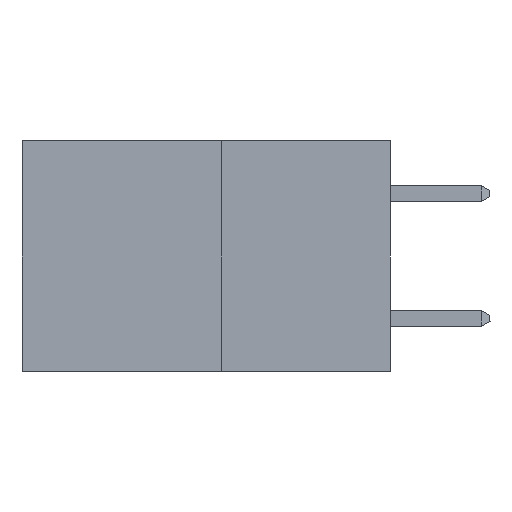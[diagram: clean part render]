
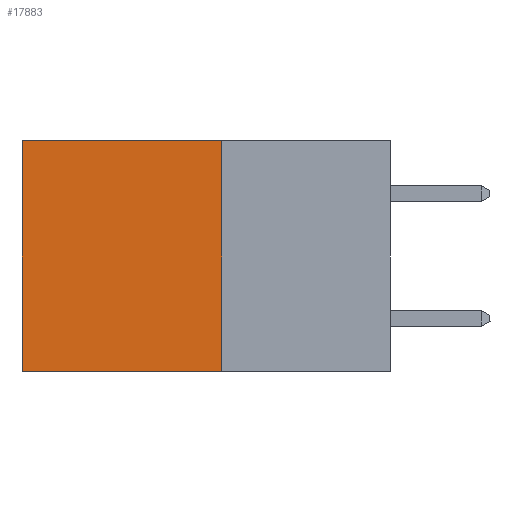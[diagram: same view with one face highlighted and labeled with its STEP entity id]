
A CAD part, left-side view. The second image highlights one B-rep face of the part: STEP entity #17883.
In plain terms, the highlighted planar face has unit normal (-1, 0, 0).
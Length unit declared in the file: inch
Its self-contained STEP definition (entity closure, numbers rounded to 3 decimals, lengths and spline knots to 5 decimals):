
#1280 = VECTOR ( 'NONE', #5275, 39.37008 ) ;
#1611 = LINE ( 'NONE', #2699, #14291 ) ;
#2421 = DIRECTION ( 'NONE',  ( 0., 0., -1. ) ) ;
#2699 = CARTESIAN_POINT ( 'NONE',  ( 0.277, 0.27, -0.37 ) ) ;
#2813 = EDGE_CURVE ( 'NONE', #3891, #9811, #1611, .T. ) ;
#3512 = EDGE_LOOP ( 'NONE', ( #18619, #8255, #10140, #17256 ) ) ;
#3551 = CARTESIAN_POINT ( 'NONE',  ( 0.277, 0.59, -0.37 ) ) ;
#3891 = VERTEX_POINT ( 'NONE', #12034 ) ;
#5121 = CARTESIAN_POINT ( 'NONE',  ( 0.277, 0.27, -0.37 ) ) ;
#5275 = DIRECTION ( 'NONE',  ( 0., 1., 0. ) ) ;
#5608 = PLANE ( 'NONE',  #21144 ) ;
#6104 = EDGE_CURVE ( 'NONE', #6262, #18843, #11326, .T. ) ;
#6262 = VERTEX_POINT ( 'NONE', #11653 ) ;
#6330 = VECTOR ( 'NONE', #8164, 39.37008 ) ;
#6882 = VECTOR ( 'NONE', #13435, 39.37008 ) ;
#8164 = DIRECTION ( 'NONE',  ( 0., 1., 0. ) ) ;
#8190 = CARTESIAN_POINT ( 'NONE',  ( 0.277, 0.27, 0. ) ) ;
#8206 = DIRECTION ( 'NONE',  ( 0., 0., -1. ) ) ;
#8219 = EDGE_CURVE ( 'NONE', #9811, #18843, #15004, .T. ) ;
#8255 = ORIENTED_EDGE ( 'NONE', *, *, #8219, .F. ) ;
#8948 = CARTESIAN_POINT ( 'NONE',  ( 0.277, 0.27, -0.37 ) ) ;
#9811 = VERTEX_POINT ( 'NONE', #14873 ) ;
#10140 = ORIENTED_EDGE ( 'NONE', *, *, #2813, .F. ) ;
#10428 = EDGE_CURVE ( 'NONE', #3891, #6262, #15190, .T. ) ;
#11326 = LINE ( 'NONE', #3551, #6882 ) ;
#11653 = CARTESIAN_POINT ( 'NONE',  ( 0.277, 0.59, 0. ) ) ;
#12034 = CARTESIAN_POINT ( 'NONE',  ( 0.277, 0.27, 0. ) ) ;
#12283 = DIRECTION ( 'NONE',  ( 1., 0., 0. ) ) ;
#13209 = CARTESIAN_POINT ( 'NONE',  ( 0.277, 0.59, -0.37 ) ) ;
#13435 = DIRECTION ( 'NONE',  ( 0., 0., -1. ) ) ;
#14291 = VECTOR ( 'NONE', #8206, 39.37008 ) ;
#14873 = CARTESIAN_POINT ( 'NONE',  ( 0.277, 0.27, -0.37 ) ) ;
#15004 = LINE ( 'NONE', #5121, #1280 ) ;
#15190 = LINE ( 'NONE', #8190, #6330 ) ;
#17256 = ORIENTED_EDGE ( 'NONE', *, *, #10428, .T. ) ;
#17883 = ADVANCED_FACE ( 'NONE', ( #18268 ), #5608, .F. ) ;
#18268 = FACE_OUTER_BOUND ( 'NONE', #3512, .T. ) ;
#18619 = ORIENTED_EDGE ( 'NONE', *, *, #6104, .T. ) ;
#18843 = VERTEX_POINT ( 'NONE', #13209 ) ;
#21144 = AXIS2_PLACEMENT_3D ( 'NONE', #8948, #12283, #2421 ) ;
